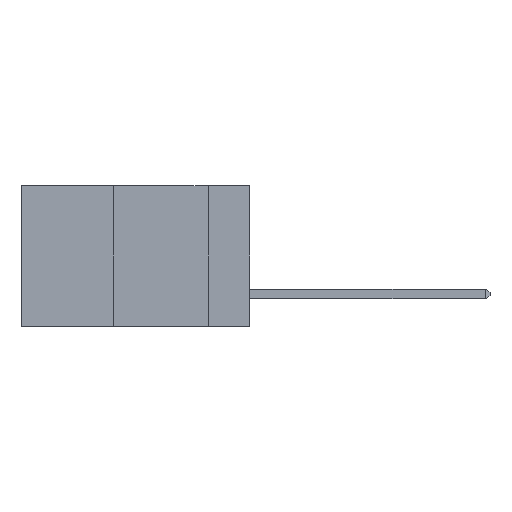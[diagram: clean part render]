
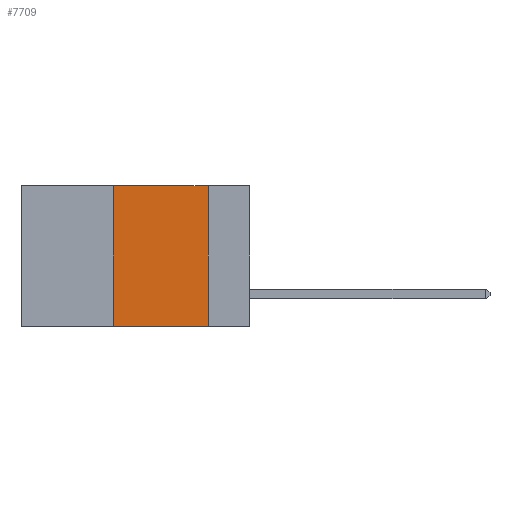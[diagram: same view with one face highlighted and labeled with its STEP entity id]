
A CAD part, left-side view. The second image highlights one B-rep face of the part: STEP entity #7709.
In plain terms, the highlighted planar face has unit normal (-1, 0, 0).
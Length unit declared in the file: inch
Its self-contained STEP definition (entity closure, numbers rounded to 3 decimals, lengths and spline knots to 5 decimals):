
#1043 = VECTOR ( 'NONE', #4872, 39.37008 ) ;
#2568 = ORIENTED_EDGE ( 'NONE', *, *, #22455, .F. ) ;
#2711 = ORIENTED_EDGE ( 'NONE', *, *, #29595, .T. ) ;
#4760 = CARTESIAN_POINT ( 'NONE',  ( 0., 0.6, 0. ) ) ;
#4788 = DIRECTION ( 'NONE',  ( 0., 0., -1. ) ) ;
#4872 = DIRECTION ( 'NONE',  ( 0., -1., 0. ) ) ;
#7709 = ADVANCED_FACE ( 'NONE', ( #21556 ), #18310, .F. ) ;
#7920 = EDGE_LOOP ( 'NONE', ( #2568, #27037, #17424, #2711 ) ) ;
#8298 = LINE ( 'NONE', #4760, #1043 ) ;
#8729 = LINE ( 'NONE', #28181, #30187 ) ;
#9176 = DIRECTION ( 'NONE',  ( 0., -1., 0. ) ) ;
#11932 = CARTESIAN_POINT ( 'NONE',  ( 0., 0.11, -0.37 ) ) ;
#13416 = VERTEX_POINT ( 'NONE', #24698 ) ;
#17424 = ORIENTED_EDGE ( 'NONE', *, *, #27820, .F. ) ;
#18310 = PLANE ( 'NONE',  #30972 ) ;
#19025 = VECTOR ( 'NONE', #29048, 39.37008 ) ;
#19853 = LINE ( 'NONE', #26367, #19025 ) ;
#20854 = VERTEX_POINT ( 'NONE', #26498 ) ;
#20966 = DIRECTION ( 'NONE',  ( 1., 0., 0. ) ) ;
#21180 = VERTEX_POINT ( 'NONE', #11932 ) ;
#21556 = FACE_OUTER_BOUND ( 'NONE', #7920, .T. ) ;
#21791 = LINE ( 'NONE', #25320, #22629 ) ;
#22455 = EDGE_CURVE ( 'NONE', #13416, #21180, #8729, .T. ) ;
#22629 = VECTOR ( 'NONE', #9176, 39.37008 ) ;
#22653 = EDGE_CURVE ( 'NONE', #20854, #13416, #8298, .T. ) ;
#24648 = VERTEX_POINT ( 'NONE', #27106 ) ;
#24698 = CARTESIAN_POINT ( 'NONE',  ( 0., 0.11, 0. ) ) ;
#25320 = CARTESIAN_POINT ( 'NONE',  ( 0., 0.6, -0.37 ) ) ;
#26367 = CARTESIAN_POINT ( 'NONE',  ( 0., 0.36, 0. ) ) ;
#26498 = CARTESIAN_POINT ( 'NONE',  ( 0., 0.36, 0. ) ) ;
#27037 = ORIENTED_EDGE ( 'NONE', *, *, #22653, .F. ) ;
#27106 = CARTESIAN_POINT ( 'NONE',  ( 0., 0.36, -0.37 ) ) ;
#27820 = EDGE_CURVE ( 'NONE', #24648, #20854, #19853, .T. ) ;
#28181 = CARTESIAN_POINT ( 'NONE',  ( 0., 0.11, 0. ) ) ;
#28888 = CARTESIAN_POINT ( 'NONE',  ( 0., 0.6, 0. ) ) ;
#29048 = DIRECTION ( 'NONE',  ( 0., 0., 1. ) ) ;
#29595 = EDGE_CURVE ( 'NONE', #24648, #21180, #21791, .T. ) ;
#30187 = VECTOR ( 'NONE', #30851, 39.37008 ) ;
#30851 = DIRECTION ( 'NONE',  ( 0., 0., -1. ) ) ;
#30972 = AXIS2_PLACEMENT_3D ( 'NONE', #28888, #20966, #4788 ) ;
